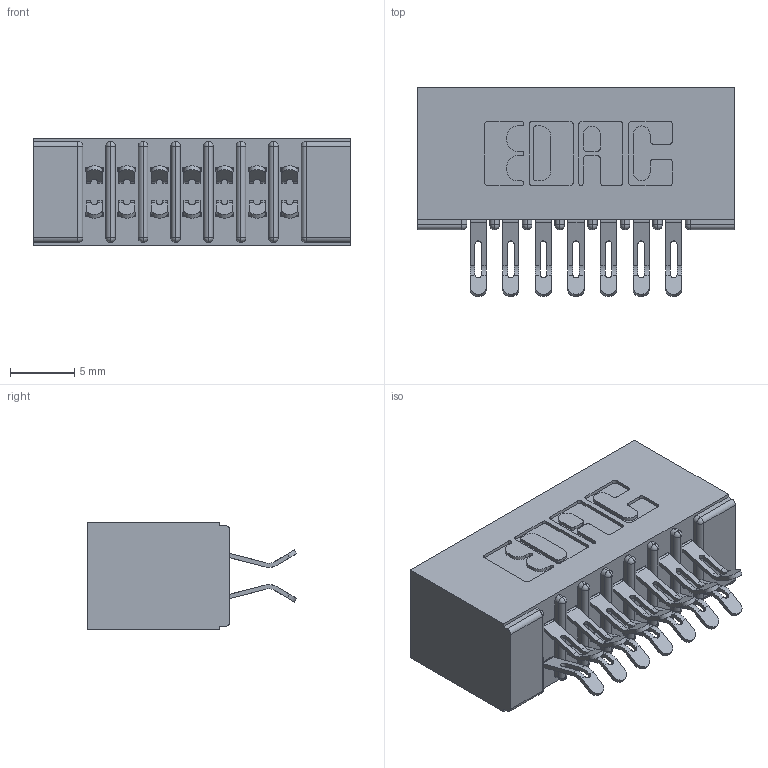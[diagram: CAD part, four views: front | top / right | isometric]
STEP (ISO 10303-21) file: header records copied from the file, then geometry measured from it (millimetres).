
FILE_DESCRIPTION (( 'STEP AP203' ), '1' );
FILE_NAME ('391-014-555-201.STEP', '2018-08-08T17:13:05', ( '' ), ( '' ), 'SwSTEP 2.0', 'SolidWorks 2016', '' );
FILE_SCHEMA (( 'CONFIG_CONTROL_DESIGN' ));
Length unit declared in the file: inch
Products named in the file (3): 341 Part_No Mounting Lugs; 341-292-001_341-292-155; 391-014-555-201
Assembly tree (15 placements, depth 2):
  391-014-555-201
    341 Part_No Mounting Lugs
    341-292-001_341-292-155  x14
Bounding box: 24.77 x 16.31 x 8.38 mm (x, y, z)
Volume: 1597.4 mm3; surface area: 3188.6 mm2
Topology: 15 solids, 15 shells, 1200 faces, 3561 edges, 2318 vertices
Faces by surface type: plane 652, cylinder 520, sphere 16, torus 12
Entity records: 13326 total; most frequent: CARTESIAN_POINT 2231, ORIENTED_EDGE 2202, DIRECTION 2179, EDGE_CURVE 1101, VECTOR 839, LINE 839, VERTEX_POINT 706, AXIS2_PLACEMENT_3D 670
